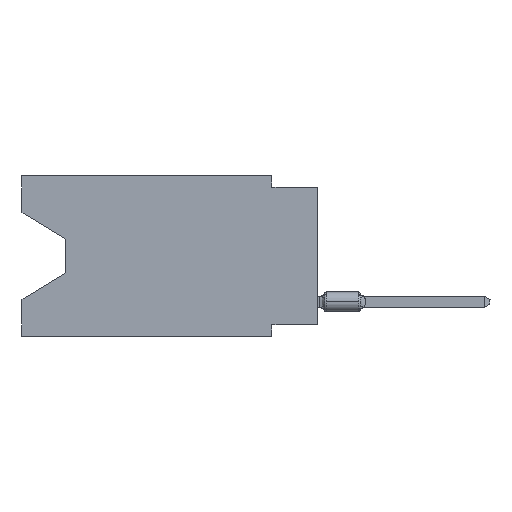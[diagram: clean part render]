
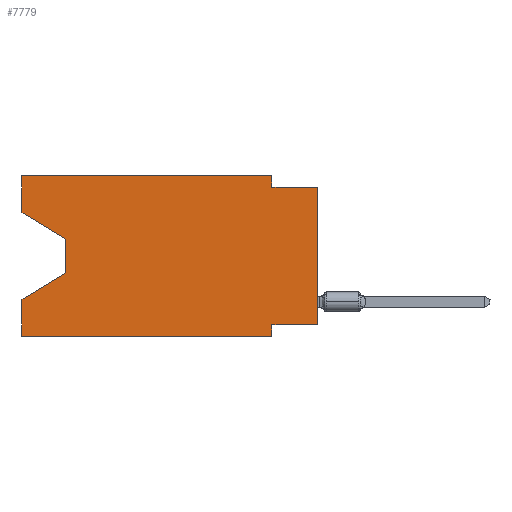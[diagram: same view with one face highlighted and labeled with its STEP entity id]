
A CAD part, left-side view. The second image highlights one B-rep face of the part: STEP entity #7779.
In plain terms, the highlighted planar face has unit normal (-1, 0, 0).
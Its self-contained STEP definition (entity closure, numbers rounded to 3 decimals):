
#1544 = CARTESIAN_POINT ( 'NONE',  ( 0., 16.383, 0. ) ) ;
#3865 = VERTEX_POINT ( 'NONE', #48366 ) ;
#4135 = DIRECTION ( 'NONE',  ( 0., 0., -1. ) ) ;
#4191 = VECTOR ( 'NONE', #69134, 1000. ) ;
#4535 = CARTESIAN_POINT ( 'NONE',  ( 0., 16.383, -8.89 ) ) ;
#4995 = LINE ( 'NONE', #11982, #94997 ) ;
#6936 = CARTESIAN_POINT ( 'NONE',  ( 0., 13.97, -3.505 ) ) ;
#7604 = VECTOR ( 'NONE', #49749, 1000. ) ;
#7773 = ORIENTED_EDGE ( 'NONE', *, *, #76925, .T. ) ;
#7779 = ADVANCED_FACE ( 'NONE', ( #70872 ), #46835, .F. ) ;
#10270 = VERTEX_POINT ( 'NONE', #17476 ) ;
#10772 = ORIENTED_EDGE ( 'NONE', *, *, #38376, .T. ) ;
#11982 = CARTESIAN_POINT ( 'NONE',  ( 0., 16.383, -2.038 ) ) ;
#12529 = CARTESIAN_POINT ( 'NONE',  ( 0., 16.383, 0. ) ) ;
#13573 = VERTEX_POINT ( 'NONE', #59458 ) ;
#13859 = EDGE_CURVE ( 'NONE', #10270, #3865, #70629, .T. ) ;
#14030 = CARTESIAN_POINT ( 'NONE',  ( 0., 0., -8.255 ) ) ;
#17476 = CARTESIAN_POINT ( 'NONE',  ( 0., 2.54, -8.255 ) ) ;
#17944 = CARTESIAN_POINT ( 'NONE',  ( 0., 16.383, -8.89 ) ) ;
#19381 = LINE ( 'NONE', #84604, #72639 ) ;
#20120 = CARTESIAN_POINT ( 'NONE',  ( 0., 2.54, 0. ) ) ;
#21185 = ORIENTED_EDGE ( 'NONE', *, *, #41230, .T. ) ;
#21416 = VERTEX_POINT ( 'NONE', #91012 ) ;
#21905 = LINE ( 'NONE', #44921, #70063 ) ;
#22439 = ORIENTED_EDGE ( 'NONE', *, *, #48411, .F. ) ;
#27833 = VERTEX_POINT ( 'NONE', #53013 ) ;
#27920 = EDGE_CURVE ( 'NONE', #32322, #51082, #19381, .T. ) ;
#28682 = VECTOR ( 'NONE', #39443, 1000. ) ;
#30266 = DIRECTION ( 'NONE',  ( 0., 0., -1. ) ) ;
#31601 = ORIENTED_EDGE ( 'NONE', *, *, #92868, .F. ) ;
#32322 = VERTEX_POINT ( 'NONE', #1544 ) ;
#36459 = ORIENTED_EDGE ( 'NONE', *, *, #73531, .T. ) ;
#37296 = CARTESIAN_POINT ( 'NONE',  ( 0., 2.54, 0. ) ) ;
#38376 = EDGE_CURVE ( 'NONE', #50480, #27833, #46141, .T. ) ;
#39443 = DIRECTION ( 'NONE',  ( 0., -1., 0. ) ) ;
#41230 = EDGE_CURVE ( 'NONE', #91331, #50480, #4995, .T. ) ;
#44921 = CARTESIAN_POINT ( 'NONE',  ( 0., 0., 0. ) ) ;
#45839 = LINE ( 'NONE', #37296, #66715 ) ;
#46141 = LINE ( 'NONE', #94763, #4191 ) ;
#46835 = PLANE ( 'NONE',  #60710 ) ;
#47828 = CARTESIAN_POINT ( 'NONE',  ( 0., 0., -8.255 ) ) ;
#48342 = LINE ( 'NONE', #47828, #60391 ) ;
#48366 = CARTESIAN_POINT ( 'NONE',  ( 0., 2.54, -8.89 ) ) ;
#48411 = EDGE_CURVE ( 'NONE', #91551, #21416, #65075, .T. ) ;
#48495 = CARTESIAN_POINT ( 'NONE',  ( 0., 0., -0.635 ) ) ;
#48944 = DIRECTION ( 'NONE',  ( 0., -1., 0. ) ) ;
#49749 = DIRECTION ( 'NONE',  ( 0., 0.855, -0.519 ) ) ;
#50480 = VERTEX_POINT ( 'NONE', #6936 ) ;
#50825 = ORIENTED_EDGE ( 'NONE', *, *, #55282, .F. ) ;
#50890 = VECTOR ( 'NONE', #92867, 1000. ) ;
#51082 = VERTEX_POINT ( 'NONE', #20120 ) ;
#53013 = CARTESIAN_POINT ( 'NONE',  ( 0., 13.97, -5.385 ) ) ;
#54732 = DIRECTION ( 'NONE',  ( 0., 0., 1. ) ) ;
#55282 = EDGE_CURVE ( 'NONE', #75422, #10270, #48342, .T. ) ;
#55817 = CARTESIAN_POINT ( 'NONE',  ( 0., 16.383, -2.038 ) ) ;
#59458 = CARTESIAN_POINT ( 'NONE',  ( 0., 16.383, -6.852 ) ) ;
#60391 = VECTOR ( 'NONE', #80446, 1000. ) ;
#60710 = AXIS2_PLACEMENT_3D ( 'NONE', #85356, #102411, #30266 ) ;
#62375 = LINE ( 'NONE', #86427, #50890 ) ;
#62528 = DIRECTION ( 'NONE',  ( 0., 0., 1. ) ) ;
#62755 = LINE ( 'NONE', #12529, #85521 ) ;
#63140 = CARTESIAN_POINT ( 'NONE',  ( 0., 2.54, -8.89 ) ) ;
#63402 = EDGE_CURVE ( 'NONE', #84765, #13573, #62375, .T. ) ;
#65075 = LINE ( 'NONE', #48495, #28682 ) ;
#65709 = VECTOR ( 'NONE', #78136, 1000. ) ;
#66488 = ORIENTED_EDGE ( 'NONE', *, *, #13859, .F. ) ;
#66715 = VECTOR ( 'NONE', #4135, 1000. ) ;
#69134 = DIRECTION ( 'NONE',  ( 0., 0., -1. ) ) ;
#70063 = VECTOR ( 'NONE', #62528, 1000. ) ;
#70200 = ORIENTED_EDGE ( 'NONE', *, *, #103024, .F. ) ;
#70629 = LINE ( 'NONE', #63140, #65709 ) ;
#70872 = FACE_OUTER_BOUND ( 'NONE', #78060, .T. ) ;
#72639 = VECTOR ( 'NONE', #101139, 1000. ) ;
#73434 = CARTESIAN_POINT ( 'NONE',  ( 0., 2.54, -0.635 ) ) ;
#73531 = EDGE_CURVE ( 'NONE', #84765, #3865, #91169, .T. ) ;
#75422 = VERTEX_POINT ( 'NONE', #14030 ) ;
#76925 = EDGE_CURVE ( 'NONE', #27833, #13573, #91971, .T. ) ;
#77459 = ORIENTED_EDGE ( 'NONE', *, *, #92518, .T. ) ;
#78060 = EDGE_LOOP ( 'NONE', ( #21185, #10772, #7773, #88223, #36459, #66488, #50825, #77459, #22439, #31601, #98817, #70200 ) ) ;
#78136 = DIRECTION ( 'NONE',  ( 0., 0., -1. ) ) ;
#80446 = DIRECTION ( 'NONE',  ( 0., 1., 0. ) ) ;
#84604 = CARTESIAN_POINT ( 'NONE',  ( 0., 16.383, 0. ) ) ;
#84716 = DIRECTION ( 'NONE',  ( 0., -0.855, -0.519 ) ) ;
#84765 = VERTEX_POINT ( 'NONE', #4535 ) ;
#85356 = CARTESIAN_POINT ( 'NONE',  ( 0., 16.383, 0. ) ) ;
#85521 = VECTOR ( 'NONE', #54732, 1000. ) ;
#86427 = CARTESIAN_POINT ( 'NONE',  ( 0., 16.383, 0. ) ) ;
#87617 = VECTOR ( 'NONE', #48944, 1000. ) ;
#88223 = ORIENTED_EDGE ( 'NONE', *, *, #63402, .F. ) ;
#90915 = CARTESIAN_POINT ( 'NONE',  ( 0., 13.97, -5.385 ) ) ;
#91012 = CARTESIAN_POINT ( 'NONE',  ( 0., 0., -0.635 ) ) ;
#91169 = LINE ( 'NONE', #17944, #87617 ) ;
#91331 = VERTEX_POINT ( 'NONE', #55817 ) ;
#91551 = VERTEX_POINT ( 'NONE', #73434 ) ;
#91971 = LINE ( 'NONE', #90915, #7604 ) ;
#92518 = EDGE_CURVE ( 'NONE', #75422, #21416, #21905, .T. ) ;
#92867 = DIRECTION ( 'NONE',  ( 0., 0., 1. ) ) ;
#92868 = EDGE_CURVE ( 'NONE', #51082, #91551, #45839, .T. ) ;
#94763 = CARTESIAN_POINT ( 'NONE',  ( 0., 13.97, -3.505 ) ) ;
#94997 = VECTOR ( 'NONE', #84716, 1000. ) ;
#98817 = ORIENTED_EDGE ( 'NONE', *, *, #27920, .F. ) ;
#101139 = DIRECTION ( 'NONE',  ( 0., -1., 0. ) ) ;
#102411 = DIRECTION ( 'NONE',  ( 1., 0., 0. ) ) ;
#103024 = EDGE_CURVE ( 'NONE', #91331, #32322, #62755, .T. ) ;
